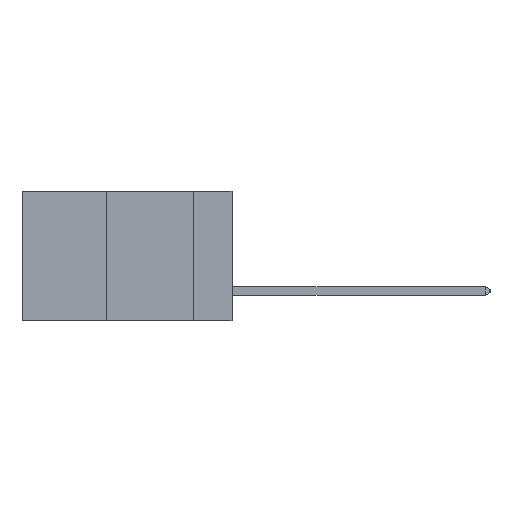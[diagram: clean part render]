
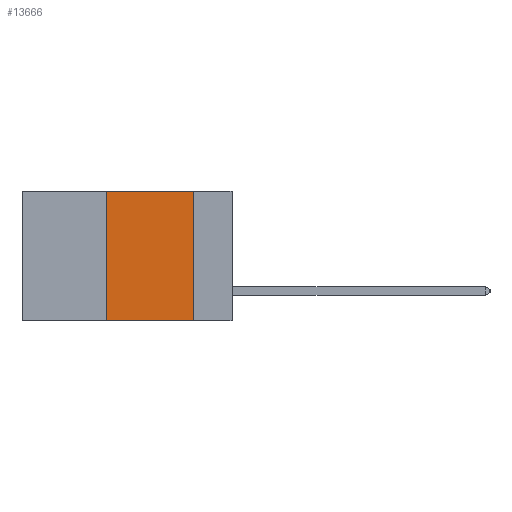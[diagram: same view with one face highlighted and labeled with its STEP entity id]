
A CAD part, left-side view. The second image highlights one B-rep face of the part: STEP entity #13666.
In plain terms, the highlighted planar face has unit normal (-1, 0, 0).
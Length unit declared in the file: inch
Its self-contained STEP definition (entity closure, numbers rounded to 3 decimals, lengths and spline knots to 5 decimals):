
#545 = VERTEX_POINT ( 'NONE', #1682 ) ;
#1682 = CARTESIAN_POINT ( 'NONE',  ( 0., 0.11, 0. ) ) ;
#3345 = VECTOR ( 'NONE', #19439, 39.37008 ) ;
#4236 = FACE_OUTER_BOUND ( 'NONE', #7077, .T. ) ;
#4447 = LINE ( 'NONE', #14417, #3345 ) ;
#4769 = VERTEX_POINT ( 'NONE', #16004 ) ;
#5286 = AXIS2_PLACEMENT_3D ( 'NONE', #7070, #18770, #9087 ) ;
#5439 = DIRECTION ( 'NONE',  ( 0., 0., 1. ) ) ;
#6285 = VERTEX_POINT ( 'NONE', #14885 ) ;
#6547 = CARTESIAN_POINT ( 'NONE',  ( 0., 0.36, 0. ) ) ;
#7070 = CARTESIAN_POINT ( 'NONE',  ( 0., 0.6, 0. ) ) ;
#7077 = EDGE_LOOP ( 'NONE', ( #20146, #7435, #11861, #17362 ) ) ;
#7435 = ORIENTED_EDGE ( 'NONE', *, *, #19143, .F. ) ;
#8256 = VECTOR ( 'NONE', #15780, 39.37008 ) ;
#9087 = DIRECTION ( 'NONE',  ( 0., 0., -1. ) ) ;
#9896 = CARTESIAN_POINT ( 'NONE',  ( 0., 0.6, -0.37 ) ) ;
#10683 = VECTOR ( 'NONE', #5439, 39.37008 ) ;
#11861 = ORIENTED_EDGE ( 'NONE', *, *, #14908, .F. ) ;
#12653 = LINE ( 'NONE', #19082, #8256 ) ;
#13666 = ADVANCED_FACE ( 'NONE', ( #4236 ), #17072, .F. ) ;
#14417 = CARTESIAN_POINT ( 'NONE',  ( 0., 0.6, 0. ) ) ;
#14885 = CARTESIAN_POINT ( 'NONE',  ( 0., 0.11, -0.37 ) ) ;
#14908 = EDGE_CURVE ( 'NONE', #4769, #18202, #19006, .T. ) ;
#15556 = CARTESIAN_POINT ( 'NONE',  ( 0., 0.36, 0. ) ) ;
#15780 = DIRECTION ( 'NONE',  ( 0., 0., -1. ) ) ;
#16004 = CARTESIAN_POINT ( 'NONE',  ( 0., 0.36, -0.37 ) ) ;
#17072 = PLANE ( 'NONE',  #5286 ) ;
#17362 = ORIENTED_EDGE ( 'NONE', *, *, #20514, .T. ) ;
#18202 = VERTEX_POINT ( 'NONE', #6547 ) ;
#18467 = LINE ( 'NONE', #9896, #21177 ) ;
#18770 = DIRECTION ( 'NONE',  ( 1., 0., 0. ) ) ;
#19006 = LINE ( 'NONE', #15556, #10683 ) ;
#19082 = CARTESIAN_POINT ( 'NONE',  ( 0., 0.11, 0. ) ) ;
#19143 = EDGE_CURVE ( 'NONE', #18202, #545, #4447, .T. ) ;
#19439 = DIRECTION ( 'NONE',  ( 0., -1., 0. ) ) ;
#19809 = DIRECTION ( 'NONE',  ( 0., -1., 0. ) ) ;
#20146 = ORIENTED_EDGE ( 'NONE', *, *, #21074, .F. ) ;
#20514 = EDGE_CURVE ( 'NONE', #4769, #6285, #18467, .T. ) ;
#21074 = EDGE_CURVE ( 'NONE', #545, #6285, #12653, .T. ) ;
#21177 = VECTOR ( 'NONE', #19809, 39.37008 ) ;
